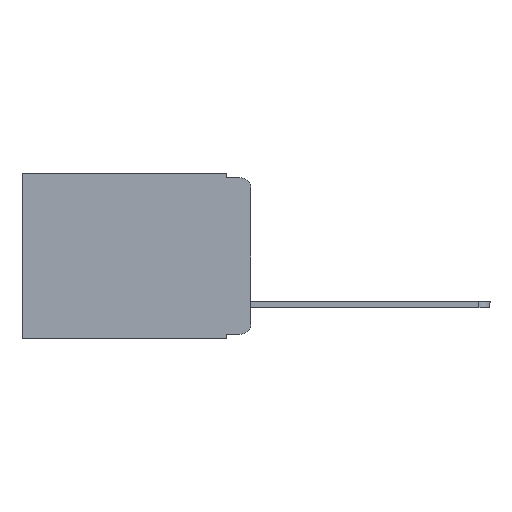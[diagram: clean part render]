
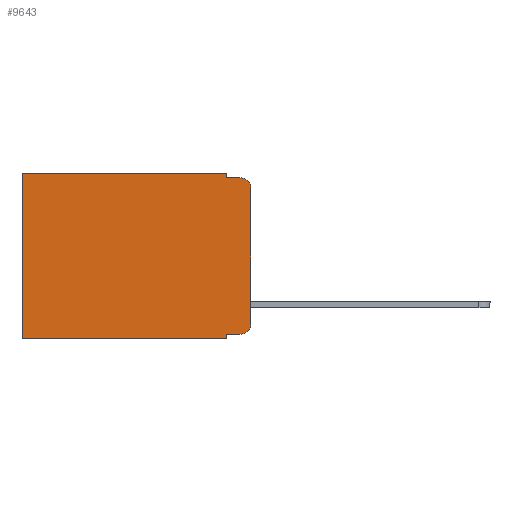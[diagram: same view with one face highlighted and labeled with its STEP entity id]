
A CAD part, left-side view. The second image highlights one B-rep face of the part: STEP entity #9643.
In plain terms, the highlighted planar face has unit normal (-1, 0, 0).
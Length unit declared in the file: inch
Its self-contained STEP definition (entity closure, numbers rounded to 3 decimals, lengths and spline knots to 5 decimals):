
#121 = CARTESIAN_POINT ( 'NONE',  ( 0.298, 0.02, -0.313 ) ) ;
#182 = CARTESIAN_POINT ( 'NONE',  ( 0.298, 0., 0. ) ) ;
#284 = EDGE_CURVE ( 'NONE', #5369, #5825, #3330, .T. ) ;
#623 = CIRCLE ( 'NONE', #6603, 0.02 ) ;
#810 = ORIENTED_EDGE ( 'NONE', *, *, #18585, .T. ) ;
#838 = CARTESIAN_POINT ( 'NONE',  ( 0.298, 0.051, -0.01 ) ) ;
#2165 = EDGE_CURVE ( 'NONE', #2570, #17241, #11185, .T. ) ;
#2237 = DIRECTION ( 'NONE',  ( 0., 0., -1. ) ) ;
#2396 = VERTEX_POINT ( 'NONE', #5455 ) ;
#2570 = VERTEX_POINT ( 'NONE', #16464 ) ;
#2750 = CARTESIAN_POINT ( 'NONE',  ( 0.298, 0.473, 0. ) ) ;
#3057 = CIRCLE ( 'NONE', #21012, 0.02 ) ;
#3173 = CARTESIAN_POINT ( 'NONE',  ( 0.298, 0., -0.343 ) ) ;
#3268 = DIRECTION ( 'NONE',  ( 0., 0., -1. ) ) ;
#3330 = LINE ( 'NONE', #8405, #3813 ) ;
#3605 = DIRECTION ( 'NONE',  ( 0., 0., -1. ) ) ;
#3617 = EDGE_CURVE ( 'NONE', #2570, #4660, #8548, .T. ) ;
#3813 = VECTOR ( 'NONE', #15995, 39.37008 ) ;
#3885 = FACE_OUTER_BOUND ( 'NONE', #16666, .T. ) ;
#4660 = VERTEX_POINT ( 'NONE', #2750 ) ;
#4719 = EDGE_CURVE ( 'NONE', #5359, #6046, #19716, .T. ) ;
#4947 = EDGE_CURVE ( 'NONE', #5369, #2396, #3057, .T. ) ;
#5359 = VERTEX_POINT ( 'NONE', #5563 ) ;
#5369 = VERTEX_POINT ( 'NONE', #12281 ) ;
#5455 = CARTESIAN_POINT ( 'NONE',  ( 0.298, 0.02, -0.01 ) ) ;
#5563 = CARTESIAN_POINT ( 'NONE',  ( 0.298, 0.051, -0.333 ) ) ;
#5777 = CARTESIAN_POINT ( 'NONE',  ( 0.298, 0.02, -0.03 ) ) ;
#5825 = VERTEX_POINT ( 'NONE', #12358 ) ;
#5872 = PLANE ( 'NONE',  #13802 ) ;
#6046 = VERTEX_POINT ( 'NONE', #17442 ) ;
#6052 = CARTESIAN_POINT ( 'NONE',  ( 0.298, 0.051, 0. ) ) ;
#6603 = AXIS2_PLACEMENT_3D ( 'NONE', #121, #11347, #10030 ) ;
#6905 = VECTOR ( 'NONE', #3268, 39.37008 ) ;
#7372 = LINE ( 'NONE', #14422, #17785 ) ;
#8098 = CARTESIAN_POINT ( 'NONE',  ( 0.298, 0.051, 0. ) ) ;
#8243 = LINE ( 'NONE', #3173, #10363 ) ;
#8405 = CARTESIAN_POINT ( 'NONE',  ( 0.298, 0., 0. ) ) ;
#8548 = LINE ( 'NONE', #182, #14468 ) ;
#8610 = ORIENTED_EDGE ( 'NONE', *, *, #14269, .F. ) ;
#8655 = DIRECTION ( 'NONE',  ( 0., 1., 0. ) ) ;
#9312 = DIRECTION ( 'NONE',  ( 0., 0., -1. ) ) ;
#9643 = ADVANCED_FACE ( 'NONE', ( #3885 ), #5872, .F. ) ;
#10007 = DIRECTION ( 'NONE',  ( 0., 1., 0. ) ) ;
#10030 = DIRECTION ( 'NONE',  ( 0., 0., -1. ) ) ;
#10363 = VECTOR ( 'NONE', #10007, 39.37008 ) ;
#10909 = CARTESIAN_POINT ( 'NONE',  ( 0.298, 0.473, -0.343 ) ) ;
#11111 = VECTOR ( 'NONE', #9312, 39.37008 ) ;
#11185 = LINE ( 'NONE', #8098, #11111 ) ;
#11335 = ORIENTED_EDGE ( 'NONE', *, *, #2165, .F. ) ;
#11347 = DIRECTION ( 'NONE',  ( -1., 0., 0. ) ) ;
#11527 = CARTESIAN_POINT ( 'NONE',  ( 0.298, 0.473, 0. ) ) ;
#12281 = CARTESIAN_POINT ( 'NONE',  ( 0.298, 0., -0.03 ) ) ;
#12358 = CARTESIAN_POINT ( 'NONE',  ( 0.298, 0., -0.313 ) ) ;
#12689 = CARTESIAN_POINT ( 'NONE',  ( 0.298, 0.051, -0.333 ) ) ;
#12930 = VECTOR ( 'NONE', #19608, 39.37008 ) ;
#13654 = DIRECTION ( 'NONE',  ( -1., 0., 0. ) ) ;
#13802 = AXIS2_PLACEMENT_3D ( 'NONE', #19320, #16127, #2237 ) ;
#13853 = VERTEX_POINT ( 'NONE', #10909 ) ;
#14269 = EDGE_CURVE ( 'NONE', #17241, #2396, #7372, .T. ) ;
#14422 = CARTESIAN_POINT ( 'NONE',  ( 0.298, 0.051, -0.01 ) ) ;
#14468 = VECTOR ( 'NONE', #8655, 39.37008 ) ;
#14557 = LINE ( 'NONE', #12689, #21735 ) ;
#14601 = ORIENTED_EDGE ( 'NONE', *, *, #17007, .F. ) ;
#15187 = ORIENTED_EDGE ( 'NONE', *, *, #3617, .T. ) ;
#15206 = EDGE_CURVE ( 'NONE', #5359, #20346, #14557, .T. ) ;
#15243 = EDGE_CURVE ( 'NONE', #20346, #5825, #623, .T. ) ;
#15995 = DIRECTION ( 'NONE',  ( 0., 0., -1. ) ) ;
#16127 = DIRECTION ( 'NONE',  ( 1., 0., 0. ) ) ;
#16464 = CARTESIAN_POINT ( 'NONE',  ( 0.298, 0.051, 0. ) ) ;
#16666 = EDGE_LOOP ( 'NONE', ( #18320, #20868, #8610, #11335, #15187, #810, #14601, #18058, #17509, #19340 ) ) ;
#16724 = LINE ( 'NONE', #11527, #6905 ) ;
#17007 = EDGE_CURVE ( 'NONE', #6046, #13853, #8243, .T. ) ;
#17241 = VERTEX_POINT ( 'NONE', #838 ) ;
#17442 = CARTESIAN_POINT ( 'NONE',  ( 0.298, 0.051, -0.343 ) ) ;
#17509 = ORIENTED_EDGE ( 'NONE', *, *, #15206, .T. ) ;
#17785 = VECTOR ( 'NONE', #17832, 39.37008 ) ;
#17832 = DIRECTION ( 'NONE',  ( 0., -1., 0. ) ) ;
#18058 = ORIENTED_EDGE ( 'NONE', *, *, #4719, .F. ) ;
#18320 = ORIENTED_EDGE ( 'NONE', *, *, #284, .F. ) ;
#18585 = EDGE_CURVE ( 'NONE', #4660, #13853, #16724, .T. ) ;
#19320 = CARTESIAN_POINT ( 'NONE',  ( 0.298, 0., 0. ) ) ;
#19340 = ORIENTED_EDGE ( 'NONE', *, *, #15243, .T. ) ;
#19608 = DIRECTION ( 'NONE',  ( 0., 0., -1. ) ) ;
#19716 = LINE ( 'NONE', #6052, #12930 ) ;
#20115 = CARTESIAN_POINT ( 'NONE',  ( 0.298, 0.02, -0.333 ) ) ;
#20346 = VERTEX_POINT ( 'NONE', #20115 ) ;
#20868 = ORIENTED_EDGE ( 'NONE', *, *, #4947, .T. ) ;
#21012 = AXIS2_PLACEMENT_3D ( 'NONE', #5777, #13654, #3605 ) ;
#21276 = DIRECTION ( 'NONE',  ( 0., -1., 0. ) ) ;
#21735 = VECTOR ( 'NONE', #21276, 39.37008 ) ;
